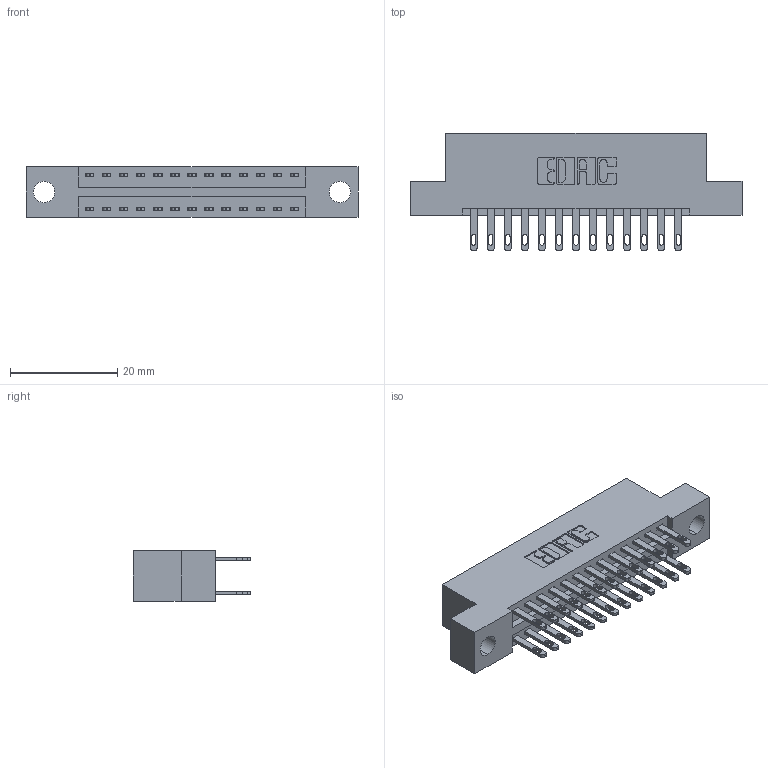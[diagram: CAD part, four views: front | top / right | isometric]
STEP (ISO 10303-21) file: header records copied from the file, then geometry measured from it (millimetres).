
FILE_DESCRIPTION (( 'STEP AP203' ), '1' );
FILE_NAME ('346-026-500-204.STEP', '2022-05-19T00:51:07', ( '' ), ( '' ), 'SwSTEP 2.0', 'SolidWorks 2020', '' );
FILE_SCHEMA (( 'CONFIG_CONTROL_DESIGN' ));
Length unit declared in the file: inch
Products named in the file (3): 346 Part_Flush Mounting Lugs - 0.156 Dia-TH; 345-292-001_345-293-100; 346-026-500-204
Assembly tree (27 placements, depth 2):
  346-026-500-204
    346 Part_Flush Mounting Lugs - 0.156 Dia-TH
    345-292-001_345-293-100  x26
Bounding box: 61.85 x 21.84 x 9.4 mm (x, y, z)
Volume: 5779.3 mm3; surface area: 7608.3 mm2
Topology: 27 solids, 27 shells, 1384 faces, 4187 edges, 2790 vertices
Faces by surface type: plane 844, cylinder 540
Entity records: 12737 total; most frequent: CARTESIAN_POINT 2142, ORIENTED_EDGE 2074, DIRECTION 1941, EDGE_CURVE 1037, LINE 849, VECTOR 849, VERTEX_POINT 690, AXIS2_PLACEMENT_3D 546
